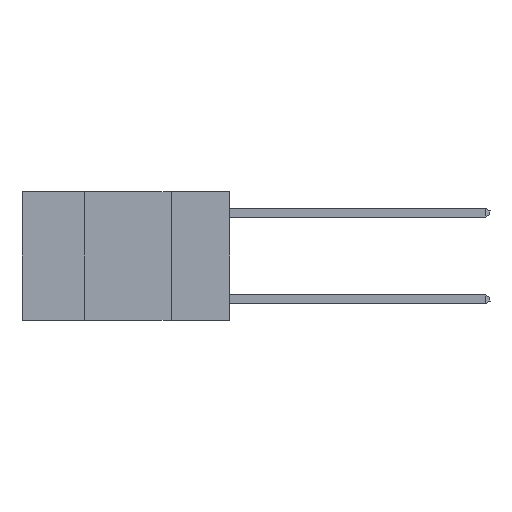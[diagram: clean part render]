
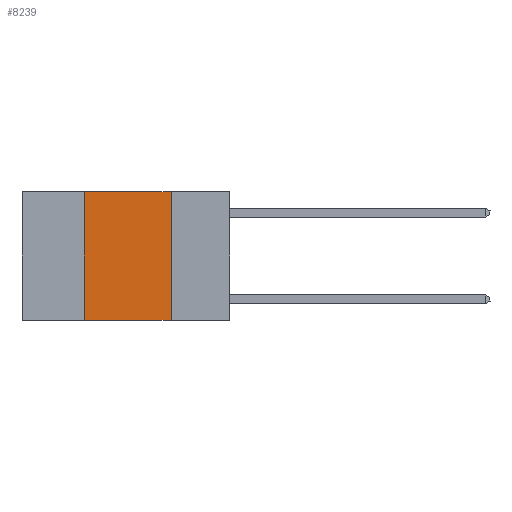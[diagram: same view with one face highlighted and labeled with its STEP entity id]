
A CAD part, left-side view. The second image highlights one B-rep face of the part: STEP entity #8239.
In plain terms, the highlighted planar face has unit normal (-1, 0, 0).
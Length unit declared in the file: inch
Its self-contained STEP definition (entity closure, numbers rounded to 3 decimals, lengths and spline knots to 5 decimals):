
#25 = VECTOR ( 'NONE', #491, 39.37008 ) ;
#421 = CARTESIAN_POINT ( 'NONE',  ( 0., 0.6, -0.37 ) ) ;
#491 = DIRECTION ( 'NONE',  ( 0., 0., -1. ) ) ;
#1176 = VERTEX_POINT ( 'NONE', #9458 ) ;
#1465 = DIRECTION ( 'NONE',  ( 0., 0., -1. ) ) ;
#1692 = VECTOR ( 'NONE', #4681, 39.37008 ) ;
#1870 = ORIENTED_EDGE ( 'NONE', *, *, #4140, .F. ) ;
#1915 = LINE ( 'NONE', #9755, #4537 ) ;
#2126 = FACE_OUTER_BOUND ( 'NONE', #7894, .T. ) ;
#3064 = CARTESIAN_POINT ( 'NONE',  ( 0., 0.6, 0. ) ) ;
#3310 = EDGE_CURVE ( 'NONE', #5656, #9391, #10404, .T. ) ;
#3321 = VERTEX_POINT ( 'NONE', #6245 ) ;
#3431 = LINE ( 'NONE', #10101, #5919 ) ;
#3521 = EDGE_CURVE ( 'NONE', #1176, #3321, #3431, .T. ) ;
#3818 = LINE ( 'NONE', #10579, #25 ) ;
#4140 = EDGE_CURVE ( 'NONE', #3321, #9391, #3818, .T. ) ;
#4537 = VECTOR ( 'NONE', #10505, 39.37008 ) ;
#4681 = DIRECTION ( 'NONE',  ( 0., -1., 0. ) ) ;
#5656 = VERTEX_POINT ( 'NONE', #9274 ) ;
#5919 = VECTOR ( 'NONE', #10238, 39.37008 ) ;
#5941 = ORIENTED_EDGE ( 'NONE', *, *, #3310, .T. ) ;
#6245 = CARTESIAN_POINT ( 'NONE',  ( 0., 0.17, 0. ) ) ;
#7111 = PLANE ( 'NONE',  #8752 ) ;
#7894 = EDGE_LOOP ( 'NONE', ( #1870, #10582, #9469, #5941 ) ) ;
#8239 = ADVANCED_FACE ( 'NONE', ( #2126 ), #7111, .F. ) ;
#8752 = AXIS2_PLACEMENT_3D ( 'NONE', #3064, #10665, #1465 ) ;
#9274 = CARTESIAN_POINT ( 'NONE',  ( 0., 0.42, -0.37 ) ) ;
#9391 = VERTEX_POINT ( 'NONE', #10645 ) ;
#9458 = CARTESIAN_POINT ( 'NONE',  ( 0., 0.42, 0. ) ) ;
#9469 = ORIENTED_EDGE ( 'NONE', *, *, #10133, .F. ) ;
#9755 = CARTESIAN_POINT ( 'NONE',  ( 0., 0.42, 0. ) ) ;
#10101 = CARTESIAN_POINT ( 'NONE',  ( 0., 0.6, 0. ) ) ;
#10133 = EDGE_CURVE ( 'NONE', #5656, #1176, #1915, .T. ) ;
#10238 = DIRECTION ( 'NONE',  ( 0., -1., 0. ) ) ;
#10404 = LINE ( 'NONE', #421, #1692 ) ;
#10505 = DIRECTION ( 'NONE',  ( 0., 0., 1. ) ) ;
#10579 = CARTESIAN_POINT ( 'NONE',  ( 0., 0.17, 0. ) ) ;
#10582 = ORIENTED_EDGE ( 'NONE', *, *, #3521, .F. ) ;
#10645 = CARTESIAN_POINT ( 'NONE',  ( 0., 0.17, -0.37 ) ) ;
#10665 = DIRECTION ( 'NONE',  ( 1., 0., 0. ) ) ;
